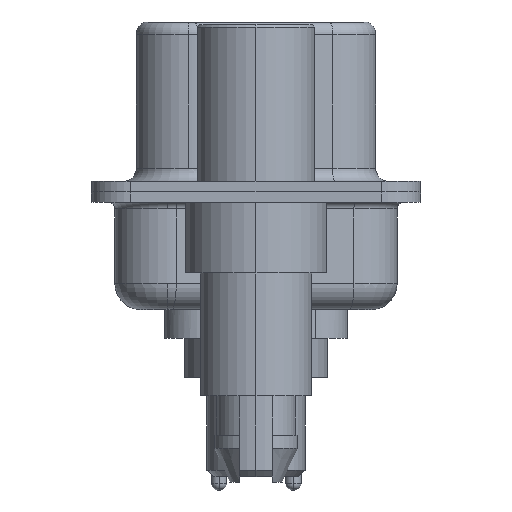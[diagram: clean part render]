
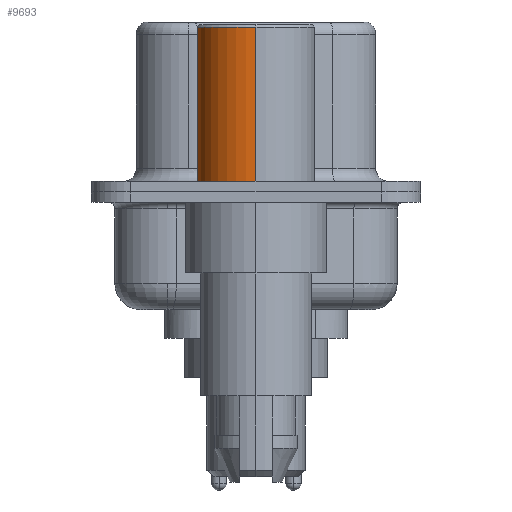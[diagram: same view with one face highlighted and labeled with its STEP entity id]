
A CAD part, left-side view. The second image highlights one B-rep face of the part: STEP entity #9693.
In plain terms, the highlighted cylindrical face has radius 2.25 mm (diameter 4.5 mm), a partial arc.
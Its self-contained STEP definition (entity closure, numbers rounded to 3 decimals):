
#283 = DIRECTION ( 'NONE',  ( 0., 0., 1. ) ) ;
#328 = DIRECTION ( 'NONE',  ( 1., 0., 0. ) ) ;
#496 = DIRECTION ( 'NONE',  ( 0., 0., 1. ) ) ;
#1198 = AXIS2_PLACEMENT_3D ( 'NONE', #16811, #283, #328 ) ;
#1276 = VERTEX_POINT ( 'NONE', #6215 ) ;
#1311 = CYLINDRICAL_SURFACE ( 'NONE', #3318, 2.25 ) ;
#2211 = LINE ( 'NONE', #12931, #12643 ) ;
#3318 = AXIS2_PLACEMENT_3D ( 'NONE', #7645, #8990, #8937 ) ;
#3627 = EDGE_CURVE ( 'NONE', #1276, #4497, #5916, .T. ) ;
#3854 = CARTESIAN_POINT ( 'NONE',  ( 2.25, 0., 0.581 ) ) ;
#4086 = ORIENTED_EDGE ( 'NONE', *, *, #12624, .F. ) ;
#4497 = VERTEX_POINT ( 'NONE', #5118 ) ;
#4669 = LINE ( 'NONE', #3854, #7894 ) ;
#4744 = DIRECTION ( 'NONE',  ( 0., 0., 1. ) ) ;
#4947 = EDGE_CURVE ( 'NONE', #10591, #9621, #9734, .T. ) ;
#5118 = CARTESIAN_POINT ( 'NONE',  ( -2.25, 0., 6.3 ) ) ;
#5916 = CIRCLE ( 'NONE', #6525, 2.25 ) ;
#6185 = FACE_OUTER_BOUND ( 'NONE', #16340, .T. ) ;
#6215 = CARTESIAN_POINT ( 'NONE',  ( 2.25, 0., 6.3 ) ) ;
#6525 = AXIS2_PLACEMENT_3D ( 'NONE', #15332, #496, #10790 ) ;
#7645 = CARTESIAN_POINT ( 'NONE',  ( 0., 0., 0.581 ) ) ;
#7894 = VECTOR ( 'NONE', #12009, 1000. ) ;
#8763 = CARTESIAN_POINT ( 'NONE',  ( -2.25, 0., 0.4 ) ) ;
#8937 = DIRECTION ( 'NONE',  ( 1., 0., 0. ) ) ;
#8990 = DIRECTION ( 'NONE',  ( 0., 0., 1. ) ) ;
#9621 = VERTEX_POINT ( 'NONE', #8763 ) ;
#9693 = ADVANCED_FACE ( 'NONE', ( #6185 ), #1311, .T. ) ;
#9734 = CIRCLE ( 'NONE', #1198, 2.25 ) ;
#10591 = VERTEX_POINT ( 'NONE', #12589 ) ;
#10790 = DIRECTION ( 'NONE',  ( 1., 0., 0. ) ) ;
#12009 = DIRECTION ( 'NONE',  ( 0., 0., 1. ) ) ;
#12589 = CARTESIAN_POINT ( 'NONE',  ( 2.25, 0., 0.4 ) ) ;
#12624 = EDGE_CURVE ( 'NONE', #10591, #1276, #4669, .T. ) ;
#12643 = VECTOR ( 'NONE', #4744, 1000. ) ;
#12931 = CARTESIAN_POINT ( 'NONE',  ( -2.25, 0., 0.581 ) ) ;
#14874 = ORIENTED_EDGE ( 'NONE', *, *, #16450, .T. ) ;
#15332 = CARTESIAN_POINT ( 'NONE',  ( 0., 0., 6.3 ) ) ;
#16067 = ORIENTED_EDGE ( 'NONE', *, *, #4947, .T. ) ;
#16340 = EDGE_LOOP ( 'NONE', ( #16067, #14874, #16918, #4086 ) ) ;
#16450 = EDGE_CURVE ( 'NONE', #9621, #4497, #2211, .T. ) ;
#16811 = CARTESIAN_POINT ( 'NONE',  ( 0., 0., 0.4 ) ) ;
#16918 = ORIENTED_EDGE ( 'NONE', *, *, #3627, .F. ) ;
